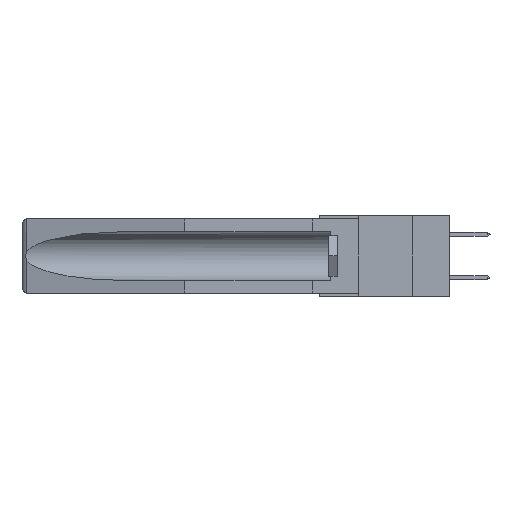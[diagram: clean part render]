
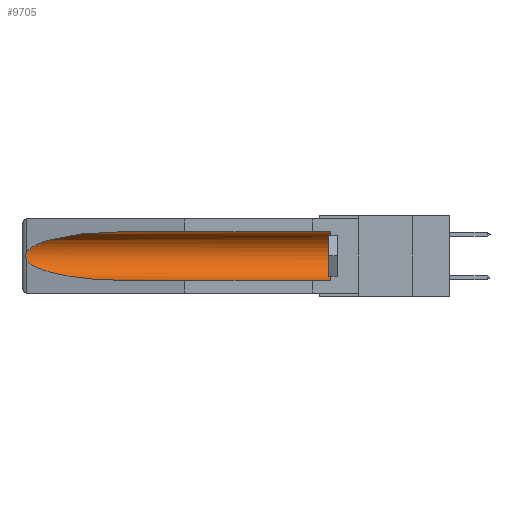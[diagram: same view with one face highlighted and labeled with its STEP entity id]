
A CAD part, left-side view. The second image highlights one B-rep face of the part: STEP entity #9705.
In plain terms, the highlighted cylindrical face has radius 2.857 mm (diameter 5.715 mm), a partial arc.
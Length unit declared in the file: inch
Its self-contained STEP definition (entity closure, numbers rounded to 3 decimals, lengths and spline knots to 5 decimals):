
#76 = CARTESIAN_POINT ( 'NONE',  ( 0.25451, 1.48313, -0.09465 ) ) ;
#361 = CARTESIAN_POINT ( 'NONE',  ( 0.26597, 1.52961, -0.15275 ) ) ;
#901 = VECTOR ( 'NONE', #10147, 39.37008 ) ;
#1075 = CARTESIAN_POINT ( 'NONE',  ( 0.155, 0.126, -0.284 ) ) ;
#1371 = VERTEX_POINT ( 'NONE', #1075 ) ;
#1573 = VERTEX_POINT ( 'NONE', #8831 ) ;
#1839 = CARTESIAN_POINT ( 'NONE',  ( 0.26537, 1.52718, -0.19328 ) ) ;
#1866 = CARTESIAN_POINT ( 'NONE',  ( 0.155, 1.07973, -0.059 ) ) ;
#2273 = VERTEX_POINT ( 'NONE', #15714 ) ;
#2788 =( BOUNDED_CURVE ( )  B_SPLINE_CURVE ( 3, ( #1866, #7558, #76, #7159 ),
 .UNSPECIFIED., .F., .T. ) 
 B_SPLINE_CURVE_WITH_KNOTS ( ( 4, 4 ),
 ( 4.71239, 6.08839 ),
 .UNSPECIFIED. ) 
 CURVE ( )  GEOMETRIC_REPRESENTATION_ITEM ( )  RATIONAL_B_SPLINE_CURVE ( ( 1., 0.848, 0.848, 1. ) ) 
 REPRESENTATION_ITEM ( '' )  );
#3197 = CARTESIAN_POINT ( 'NONE',  ( 0.2673, 1.5327, -0.16383 ) ) ;
#3538 = VECTOR ( 'NONE', #9649, 39.37008 ) ;
#3548 = EDGE_CURVE ( 'NONE', #13573, #1573, #6240, .T. ) ;
#3571 = VERTEX_POINT ( 'NONE', #13118 ) ;
#3610 = EDGE_CURVE ( 'NONE', #1573, #7861, #2788, .T. ) ;
#4389 = CARTESIAN_POINT ( 'NONE',  ( 0.21114, 1.30732, -0.284 ) ) ;
#4647 = CARTESIAN_POINT ( 'NONE',  ( 0.26597, 1.5296, -0.19026 ) ) ;
#4819 = AXIS2_PLACEMENT_3D ( 'NONE', #10567, #13441, #16570 ) ;
#5178 = ORIENTED_EDGE ( 'NONE', *, *, #8954, .T. ) ;
#5269 = ORIENTED_EDGE ( 'NONE', *, *, #3548, .T. ) ;
#5698 = CARTESIAN_POINT ( 'NONE',  ( 0.155, 1.07973, -0.284 ) ) ;
#5737 = DIRECTION ( 'NONE',  ( 0., -1., 0. ) ) ;
#5950 = CARTESIAN_POINT ( 'NONE',  ( 0.26654, 1.53092, -0.15636 ) ) ;
#6240 = LINE ( 'NONE', #16285, #3538 ) ;
#7119 = CARTESIAN_POINT ( 'NONE',  ( 0.155, 0.126, -0.1715 ) ) ;
#7159 = CARTESIAN_POINT ( 'NONE',  ( 0.26537, 1.52718, -0.14972 ) ) ;
#7212 = CIRCLE ( 'NONE', #7362, 0.1125 ) ;
#7362 = AXIS2_PLACEMENT_3D ( 'NONE', #7119, #5737, #17197 ) ;
#7466 = CARTESIAN_POINT ( 'NONE',  ( 0.26537, 1.52718, -0.14972 ) ) ;
#7558 = CARTESIAN_POINT ( 'NONE',  ( 0.21114, 1.30732, -0.059 ) ) ;
#7861 = VERTEX_POINT ( 'NONE', #12820 ) ;
#8465 = LINE ( 'NONE', #10353, #901 ) ;
#8693 = ORIENTED_EDGE ( 'NONE', *, *, #16604, .T. ) ;
#8813 = CARTESIAN_POINT ( 'NONE',  ( 0.2675, 1.53308, -0.17534 ) ) ;
#8831 = CARTESIAN_POINT ( 'NONE',  ( 0.155, 1.07973, -0.059 ) ) ;
#8954 = EDGE_CURVE ( 'NONE', #7861, #2273, #12250, .T. ) ;
#9649 = DIRECTION ( 'NONE',  ( 0., 1., 0. ) ) ;
#9705 = ADVANCED_FACE ( 'NONE', ( #17380 ), #16298, .F. ) ;
#9909 = EDGE_LOOP ( 'NONE', ( #12532, #5178, #8693, #17779, #12554, #5269 ) ) ;
#9929 = CARTESIAN_POINT ( 'NONE',  ( 0.26537, 1.52718, -0.19328 ) ) ;
#10147 = DIRECTION ( 'NONE',  ( 0., 1., 0. ) ) ;
#10196 = CARTESIAN_POINT ( 'NONE',  ( 0.2675, 1.53308, -0.16763 ) ) ;
#10353 = CARTESIAN_POINT ( 'NONE',  ( 0.155, -0.30754, -0.284 ) ) ;
#10567 = CARTESIAN_POINT ( 'NONE',  ( 0.155, -0.30754, -0.1715 ) ) ;
#12250 = B_SPLINE_CURVE_WITH_KNOTS ( 'NONE', 3,
 ( #7466, #361, #5950, #3197, #10196, #8813, #16227, #13199, #4647, #1839 ),
 .UNSPECIFIED., .F., .F.,
 ( 4, 2, 2, 2, 4 ),
 ( 0., 0.00029, 0.00058, 0.00087, 0.00117 ),
 .UNSPECIFIED. ) ;
#12440 = EDGE_CURVE ( 'NONE', #1371, #13573, #7212, .T. ) ;
#12532 = ORIENTED_EDGE ( 'NONE', *, *, #3610, .T. ) ;
#12554 = ORIENTED_EDGE ( 'NONE', *, *, #12440, .T. ) ;
#12820 = CARTESIAN_POINT ( 'NONE',  ( 0.26537, 1.52718, -0.14972 ) ) ;
#13118 = CARTESIAN_POINT ( 'NONE',  ( 0.155, 1.07973, -0.284 ) ) ;
#13199 = CARTESIAN_POINT ( 'NONE',  ( 0.26655, 1.53094, -0.18657 ) ) ;
#13441 = DIRECTION ( 'NONE',  ( 0., 1., 0. ) ) ;
#13573 = VERTEX_POINT ( 'NONE', #16628 ) ;
#14448 =( BOUNDED_CURVE ( )  B_SPLINE_CURVE ( 3, ( #9929, #15854, #4389, #5698 ),
 .UNSPECIFIED., .F., .F. ) 
 B_SPLINE_CURVE_WITH_KNOTS ( ( 4, 4 ),
 ( 0.1948, 1.5708 ),
 .UNSPECIFIED. ) 
 CURVE ( )  GEOMETRIC_REPRESENTATION_ITEM ( )  RATIONAL_B_SPLINE_CURVE ( ( 1., 0.848, 0.848, 1. ) ) 
 REPRESENTATION_ITEM ( '' )  );
#15714 = CARTESIAN_POINT ( 'NONE',  ( 0.26537, 1.52718, -0.19328 ) ) ;
#15854 = CARTESIAN_POINT ( 'NONE',  ( 0.25451, 1.48313, -0.24835 ) ) ;
#16021 = EDGE_CURVE ( 'NONE', #1371, #3571, #8465, .T. ) ;
#16227 = CARTESIAN_POINT ( 'NONE',  ( 0.2673, 1.53269, -0.17917 ) ) ;
#16285 = CARTESIAN_POINT ( 'NONE',  ( 0.155, -0.30754, -0.059 ) ) ;
#16298 = CYLINDRICAL_SURFACE ( 'NONE', #4819, 0.1125 ) ;
#16570 = DIRECTION ( 'NONE',  ( 0., 0., 1. ) ) ;
#16604 = EDGE_CURVE ( 'NONE', #2273, #3571, #14448, .T. ) ;
#16628 = CARTESIAN_POINT ( 'NONE',  ( 0.155, 0.126, -0.059 ) ) ;
#17197 = DIRECTION ( 'NONE',  ( 0., 0., 1. ) ) ;
#17380 = FACE_OUTER_BOUND ( 'NONE', #9909, .T. ) ;
#17779 = ORIENTED_EDGE ( 'NONE', *, *, #16021, .F. ) ;
